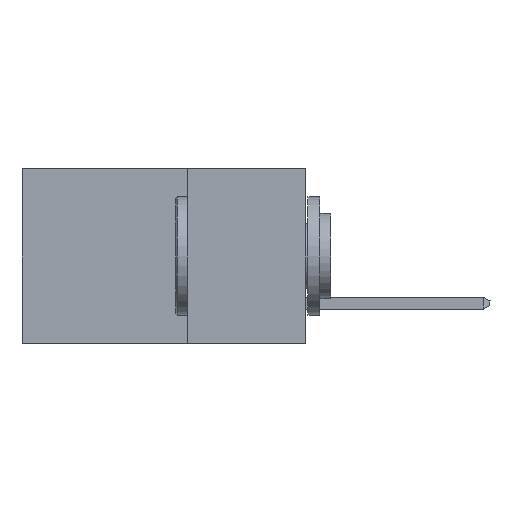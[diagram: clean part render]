
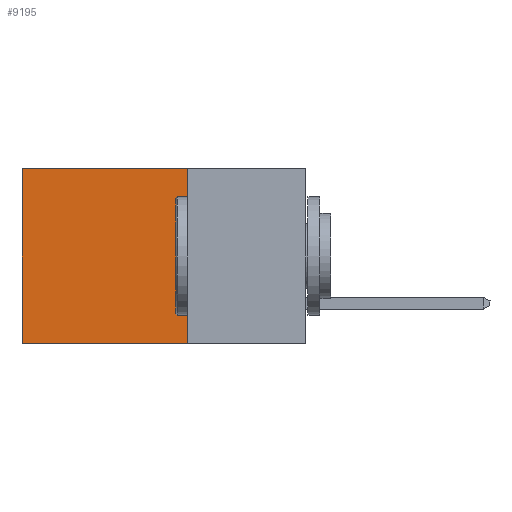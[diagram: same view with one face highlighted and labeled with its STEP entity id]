
A CAD part, left-side view. The second image highlights one B-rep face of the part: STEP entity #9195.
In plain terms, the highlighted planar face has unit normal (-1, 0, 0).
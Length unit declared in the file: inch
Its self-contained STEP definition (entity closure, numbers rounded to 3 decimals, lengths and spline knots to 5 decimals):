
#153 = DIRECTION ( 'NONE',  ( 0., 1., 0. ) ) ;
#186 = EDGE_CURVE ( 'NONE', #5934, #2661, #6981, .T. ) ;
#530 = AXIS2_PLACEMENT_3D ( 'NONE', #2717, #4891, #6281 ) ;
#625 = ORIENTED_EDGE ( 'NONE', *, *, #3442, .F. ) ;
#966 = VECTOR ( 'NONE', #6214, 39.37008 ) ;
#1018 = CARTESIAN_POINT ( 'NONE',  ( 0.2615, 0.6, -0.37 ) ) ;
#1418 = CARTESIAN_POINT ( 'NONE',  ( 0.2615, 0.25, 0. ) ) ;
#1710 = CARTESIAN_POINT ( 'NONE',  ( 0.2615, 0.6, 0. ) ) ;
#1948 = FACE_OUTER_BOUND ( 'NONE', #3941, .T. ) ;
#2119 = CARTESIAN_POINT ( 'NONE',  ( 0.2615, 0.25, -0.37 ) ) ;
#2273 = VECTOR ( 'NONE', #2401, 39.37008 ) ;
#2401 = DIRECTION ( 'NONE',  ( 0., 0., -1. ) ) ;
#2661 = VERTEX_POINT ( 'NONE', #3334 ) ;
#2717 = CARTESIAN_POINT ( 'NONE',  ( 0.2615, 0.25, -0.37 ) ) ;
#3013 = DIRECTION ( 'NONE',  ( 0., 1., 0. ) ) ;
#3334 = CARTESIAN_POINT ( 'NONE',  ( 0.2615, 0.6, -0.37 ) ) ;
#3340 = PLANE ( 'NONE',  #530 ) ;
#3442 = EDGE_CURVE ( 'NONE', #7550, #5727, #4567, .T. ) ;
#3777 = LINE ( 'NONE', #4465, #4034 ) ;
#3941 = EDGE_LOOP ( 'NONE', ( #4942, #8038, #625, #9288 ) ) ;
#4034 = VECTOR ( 'NONE', #3013, 39.37008 ) ;
#4465 = CARTESIAN_POINT ( 'NONE',  ( 0.2615, 0.25, 0. ) ) ;
#4567 = LINE ( 'NONE', #7505, #2273 ) ;
#4670 = CARTESIAN_POINT ( 'NONE',  ( 0.2615, 0.25, -0.37 ) ) ;
#4891 = DIRECTION ( 'NONE',  ( 1., 0., 0. ) ) ;
#4942 = ORIENTED_EDGE ( 'NONE', *, *, #186, .T. ) ;
#5451 = LINE ( 'NONE', #4670, #6969 ) ;
#5727 = VERTEX_POINT ( 'NONE', #2119 ) ;
#5934 = VERTEX_POINT ( 'NONE', #1710 ) ;
#6214 = DIRECTION ( 'NONE',  ( 0., 0., -1. ) ) ;
#6281 = DIRECTION ( 'NONE',  ( 0., 0., -1. ) ) ;
#6969 = VECTOR ( 'NONE', #153, 39.37008 ) ;
#6981 = LINE ( 'NONE', #1018, #966 ) ;
#7505 = CARTESIAN_POINT ( 'NONE',  ( 0.2615, 0.25, -0.37 ) ) ;
#7550 = VERTEX_POINT ( 'NONE', #1418 ) ;
#8038 = ORIENTED_EDGE ( 'NONE', *, *, #8490, .F. ) ;
#8490 = EDGE_CURVE ( 'NONE', #5727, #2661, #5451, .T. ) ;
#8727 = EDGE_CURVE ( 'NONE', #7550, #5934, #3777, .T. ) ;
#9195 = ADVANCED_FACE ( 'NONE', ( #1948 ), #3340, .F. ) ;
#9288 = ORIENTED_EDGE ( 'NONE', *, *, #8727, .T. ) ;
